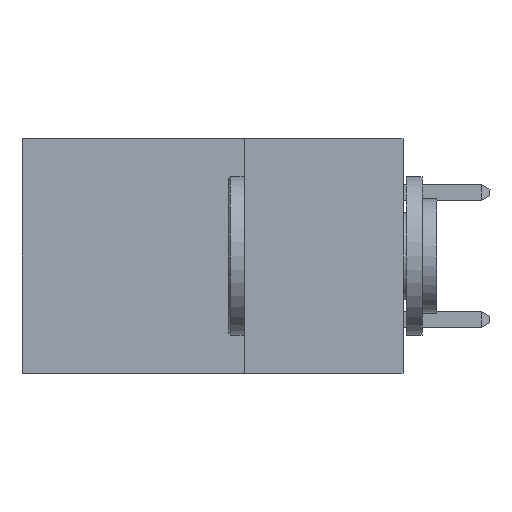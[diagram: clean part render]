
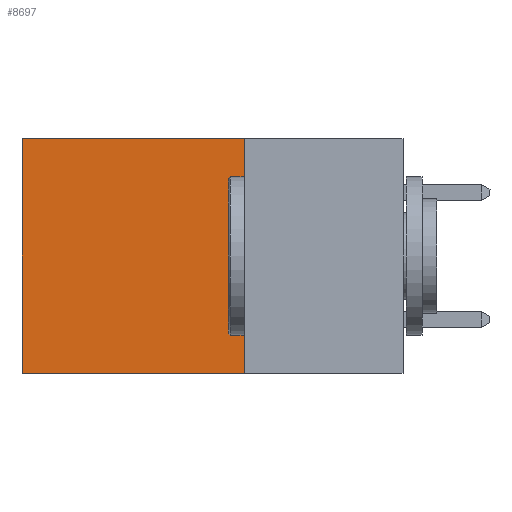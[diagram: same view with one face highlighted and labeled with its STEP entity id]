
A CAD part, left-side view. The second image highlights one B-rep face of the part: STEP entity #8697.
In plain terms, the highlighted planar face has unit normal (-1, 0, 0).
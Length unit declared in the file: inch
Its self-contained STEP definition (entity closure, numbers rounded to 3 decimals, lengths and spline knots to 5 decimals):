
#87 = DIRECTION ( 'NONE',  ( 0., 1., 0. ) ) ;
#871 = CARTESIAN_POINT ( 'NONE',  ( 0.2875, 0.25, -0.37 ) ) ;
#912 = ORIENTED_EDGE ( 'NONE', *, *, #5827, .T. ) ;
#1097 = VERTEX_POINT ( 'NONE', #7523 ) ;
#1245 = EDGE_CURVE ( 'NONE', #8933, #2445, #13114, .T. ) ;
#1639 = VECTOR ( 'NONE', #13622, 39.37008 ) ;
#2445 = VERTEX_POINT ( 'NONE', #871 ) ;
#3338 = DIRECTION ( 'NONE',  ( 0., 0., -1. ) ) ;
#3483 = ORIENTED_EDGE ( 'NONE', *, *, #14022, .F. ) ;
#3691 = VECTOR ( 'NONE', #14135, 39.37008 ) ;
#3988 = CARTESIAN_POINT ( 'NONE',  ( 0.2875, 0.6, 0. ) ) ;
#4272 = CARTESIAN_POINT ( 'NONE',  ( 0.2875, 0.25, 0. ) ) ;
#4361 = EDGE_CURVE ( 'NONE', #10188, #1097, #13044, .T. ) ;
#4810 = EDGE_LOOP ( 'NONE', ( #13477, #3483, #14219, #912 ) ) ;
#5827 = EDGE_CURVE ( 'NONE', #8933, #10188, #8471, .T. ) ;
#6536 = FACE_OUTER_BOUND ( 'NONE', #4810, .T. ) ;
#7523 = CARTESIAN_POINT ( 'NONE',  ( 0.2875, 0.6, -0.37 ) ) ;
#8157 = PLANE ( 'NONE',  #10554 ) ;
#8471 = LINE ( 'NONE', #4272, #1639 ) ;
#8697 = ADVANCED_FACE ( 'NONE', ( #6536 ), #8157, .F. ) ;
#8879 = LINE ( 'NONE', #13235, #14327 ) ;
#8933 = VERTEX_POINT ( 'NONE', #13203 ) ;
#9337 = CARTESIAN_POINT ( 'NONE',  ( 0.2875, 0.25, 0. ) ) ;
#10188 = VERTEX_POINT ( 'NONE', #3988 ) ;
#10484 = DIRECTION ( 'NONE',  ( 1., 0., 0. ) ) ;
#10554 = AXIS2_PLACEMENT_3D ( 'NONE', #9337, #10484, #3338 ) ;
#13044 = LINE ( 'NONE', #14393, #15387 ) ;
#13114 = LINE ( 'NONE', #14105, #3691 ) ;
#13203 = CARTESIAN_POINT ( 'NONE',  ( 0.2875, 0.25, 0. ) ) ;
#13235 = CARTESIAN_POINT ( 'NONE',  ( 0.2875, 0.25, -0.37 ) ) ;
#13477 = ORIENTED_EDGE ( 'NONE', *, *, #4361, .T. ) ;
#13622 = DIRECTION ( 'NONE',  ( 0., 1., 0. ) ) ;
#14022 = EDGE_CURVE ( 'NONE', #2445, #1097, #8879, .T. ) ;
#14105 = CARTESIAN_POINT ( 'NONE',  ( 0.2875, 0.25, 0. ) ) ;
#14135 = DIRECTION ( 'NONE',  ( 0., 0., -1. ) ) ;
#14219 = ORIENTED_EDGE ( 'NONE', *, *, #1245, .F. ) ;
#14327 = VECTOR ( 'NONE', #87, 39.37008 ) ;
#14393 = CARTESIAN_POINT ( 'NONE',  ( 0.2875, 0.6, 0. ) ) ;
#15338 = DIRECTION ( 'NONE',  ( 0., 0., -1. ) ) ;
#15387 = VECTOR ( 'NONE', #15338, 39.37008 ) ;
